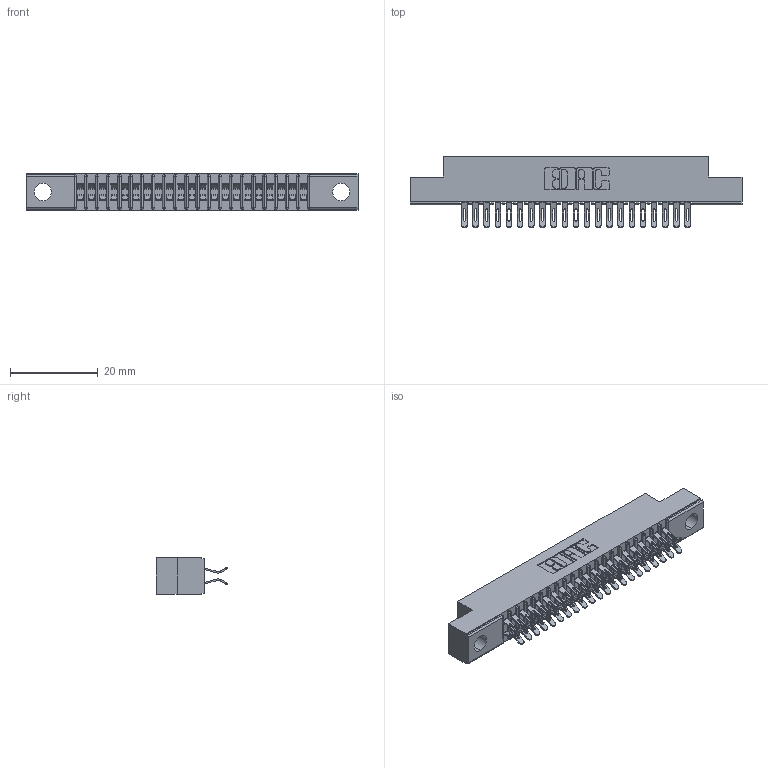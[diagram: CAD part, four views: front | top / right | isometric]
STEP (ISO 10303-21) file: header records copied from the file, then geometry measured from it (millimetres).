
FILE_DESCRIPTION (( 'STEP AP203' ), '1' );
FILE_NAME ('391-042-555-204.STEP', '2018-08-09T01:52:03', ( '' ), ( '' ), 'SwSTEP 2.0', 'SolidWorks 2016', '' );
FILE_SCHEMA (( 'CONFIG_CONTROL_DESIGN' ));
Length unit declared in the file: inch
Products named in the file (3): 341 Part_.156 (3.96) Dia Mounting Holes; 341-292-001_341-292-155; 391-042-555-204
Assembly tree (43 placements, depth 2):
  391-042-555-204
    341 Part_.156 (3.96) Dia Mounting Holes
    341-292-001_341-292-155  x42
Bounding box: 75.56 x 16.31 x 8.38 mm (x, y, z)
Volume: 4252.2 mm3; surface area: 9040 mm2
Topology: 43 solids, 43 shells, 3406 faces, 10159 edges, 6614 vertices
Faces by surface type: plane 1846, cylinder 1476, sphere 44, torus 40
Entity records: 29100 total; most frequent: CARTESIAN_POINT 4859, ORIENTED_EDGE 4814, DIRECTION 4713, EDGE_CURVE 2407, LINE 1913, VECTOR 1913, VERTEX_POINT 1530, AXIS2_PLACEMENT_3D 1400
